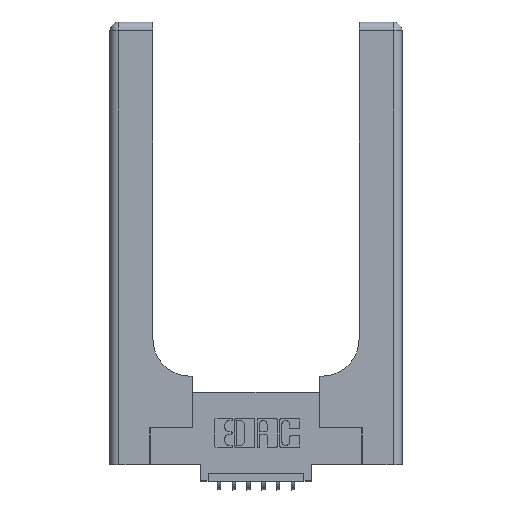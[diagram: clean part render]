
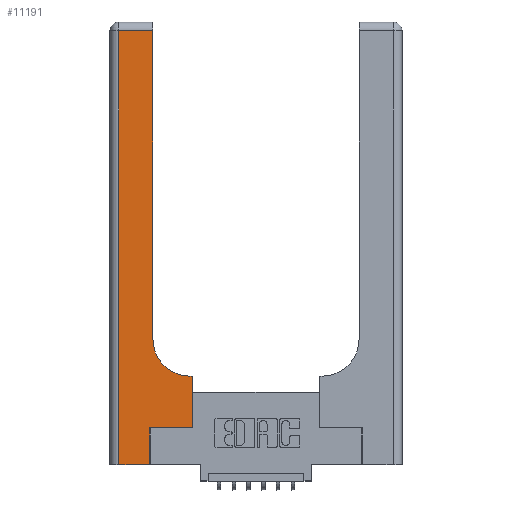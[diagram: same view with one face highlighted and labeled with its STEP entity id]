
A CAD part, top view. The second image highlights one B-rep face of the part: STEP entity #11191.
In plain terms, the highlighted planar face has unit normal (0, 0, 1).
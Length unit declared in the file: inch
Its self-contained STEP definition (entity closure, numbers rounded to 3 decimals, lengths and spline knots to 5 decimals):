
#6 = CARTESIAN_POINT ( 'NONE',  ( 0.5585, 0.6, 0.37 ) ) ;
#10 = DIRECTION ( 'NONE',  ( -1., 0., 0. ) ) ;
#196 = LINE ( 'NONE', #6288, #8931 ) ;
#241 = VECTOR ( 'NONE', #11092, 39.37008 ) ;
#779 = CARTESIAN_POINT ( 'NONE',  ( 0., 2.94, 0.37 ) ) ;
#881 = VERTEX_POINT ( 'NONE', #7257 ) ;
#1211 = DIRECTION ( 'NONE',  ( 0., 1., 0. ) ) ;
#1300 = AXIS2_PLACEMENT_3D ( 'NONE', #3464, #9089, #12483 ) ;
#1366 = CIRCLE ( 'NONE', #3056, 0.25 ) ;
#1605 = CARTESIAN_POINT ( 'NONE',  ( 0.06, 0., 0.37 ) ) ;
#1999 = ORIENTED_EDGE ( 'NONE', *, *, #5809, .T. ) ;
#2008 = VERTEX_POINT ( 'NONE', #1605 ) ;
#2251 = LINE ( 'NONE', #779, #14726 ) ;
#2322 = PLANE ( 'NONE',  #1300 ) ;
#2616 = LINE ( 'NONE', #11241, #3120 ) ;
#3010 = VERTEX_POINT ( 'NONE', #11659 ) ;
#3021 = EDGE_CURVE ( 'NONE', #881, #8735, #1366, .T. ) ;
#3056 = AXIS2_PLACEMENT_3D ( 'NONE', #10377, #7091, #3513 ) ;
#3120 = VECTOR ( 'NONE', #10, 39.37008 ) ;
#3332 = VECTOR ( 'NONE', #9706, 39.37008 ) ;
#3464 = CARTESIAN_POINT ( 'NONE',  ( 0., 3., 0.37 ) ) ;
#3513 = DIRECTION ( 'NONE',  ( 1., 0., 0. ) ) ;
#3998 = ORIENTED_EDGE ( 'NONE', *, *, #12909, .T. ) ;
#4197 = VECTOR ( 'NONE', #4644, 39.37008 ) ;
#4644 = DIRECTION ( 'NONE',  ( 0., 1., 0. ) ) ;
#4734 = LINE ( 'NONE', #7146, #4197 ) ;
#4872 = ORIENTED_EDGE ( 'NONE', *, *, #13298, .T. ) ;
#5085 = CARTESIAN_POINT ( 'NONE',  ( 0.2915, 2.94, 0.37 ) ) ;
#5089 = VECTOR ( 'NONE', #1211, 39.37008 ) ;
#5194 = ORIENTED_EDGE ( 'NONE', *, *, #3021, .T. ) ;
#5609 = EDGE_CURVE ( 'NONE', #2008, #5662, #13123, .T. ) ;
#5662 = VERTEX_POINT ( 'NONE', #8996 ) ;
#5809 = EDGE_CURVE ( 'NONE', #14651, #7820, #4734, .T. ) ;
#5838 = CARTESIAN_POINT ( 'NONE',  ( 0.2915, 3., 0.37 ) ) ;
#6124 = CARTESIAN_POINT ( 'NONE',  ( 0.5585, 0.25, 0.37 ) ) ;
#6288 = CARTESIAN_POINT ( 'NONE',  ( 0.269, 0.25, 0.37 ) ) ;
#6481 = ORIENTED_EDGE ( 'NONE', *, *, #12152, .T. ) ;
#7091 = DIRECTION ( 'NONE',  ( 0., 0., -1. ) ) ;
#7146 = CARTESIAN_POINT ( 'NONE',  ( 0.5585, 0.25, 0.37 ) ) ;
#7211 = ORIENTED_EDGE ( 'NONE', *, *, #9354, .T. ) ;
#7257 = CARTESIAN_POINT ( 'NONE',  ( 0.5415, 0.6, 0.37 ) ) ;
#7291 = EDGE_LOOP ( 'NONE', ( #6481, #7211, #8939, #11789, #4872, #3998, #1999, #8598, #5194 ) ) ;
#7618 = CARTESIAN_POINT ( 'NONE',  ( 0.2915, 0.85, 0.37 ) ) ;
#7820 = VERTEX_POINT ( 'NONE', #6 ) ;
#8059 = EDGE_CURVE ( 'NONE', #3010, #2008, #8874, .T. ) ;
#8087 = LINE ( 'NONE', #5838, #5089 ) ;
#8432 = CARTESIAN_POINT ( 'NONE',  ( 0.06, 3., 0.37 ) ) ;
#8598 = ORIENTED_EDGE ( 'NONE', *, *, #10104, .T. ) ;
#8645 = FACE_OUTER_BOUND ( 'NONE', #7291, .T. ) ;
#8735 = VERTEX_POINT ( 'NONE', #7618 ) ;
#8792 = CARTESIAN_POINT ( 'NONE',  ( 0., 0., 0.37 ) ) ;
#8815 = DIRECTION ( 'NONE',  ( -1., 0., 0. ) ) ;
#8874 = LINE ( 'NONE', #8432, #3332 ) ;
#8931 = VECTOR ( 'NONE', #9494, 39.37008 ) ;
#8939 = ORIENTED_EDGE ( 'NONE', *, *, #8059, .T. ) ;
#8996 = CARTESIAN_POINT ( 'NONE',  ( 0.269, 0., 0.37 ) ) ;
#9089 = DIRECTION ( 'NONE',  ( 0., 0., -1. ) ) ;
#9354 = EDGE_CURVE ( 'NONE', #13551, #3010, #2251, .T. ) ;
#9379 = CARTESIAN_POINT ( 'NONE',  ( 0.269, 0., 0.37 ) ) ;
#9494 = DIRECTION ( 'NONE',  ( 1., 0., 0. ) ) ;
#9706 = DIRECTION ( 'NONE',  ( 0., -1., 0. ) ) ;
#9979 = CARTESIAN_POINT ( 'NONE',  ( 0.269, 0.25, 0.37 ) ) ;
#10104 = EDGE_CURVE ( 'NONE', #7820, #881, #2616, .T. ) ;
#10377 = CARTESIAN_POINT ( 'NONE',  ( 0.5415, 0.85, 0.37 ) ) ;
#11092 = DIRECTION ( 'NONE',  ( 1., 0., 0. ) ) ;
#11191 = ADVANCED_FACE ( 'NONE', ( #8645 ), #2322, .F. ) ;
#11241 = CARTESIAN_POINT ( 'NONE',  ( 0.2915, 0.6, 0.37 ) ) ;
#11527 = DIRECTION ( 'NONE',  ( 0., 1., 0. ) ) ;
#11622 = LINE ( 'NONE', #9379, #13754 ) ;
#11659 = CARTESIAN_POINT ( 'NONE',  ( 0.06, 2.94, 0.37 ) ) ;
#11789 = ORIENTED_EDGE ( 'NONE', *, *, #5609, .T. ) ;
#12054 = VERTEX_POINT ( 'NONE', #9979 ) ;
#12152 = EDGE_CURVE ( 'NONE', #8735, #13551, #8087, .T. ) ;
#12483 = DIRECTION ( 'NONE',  ( -1., 0., 0. ) ) ;
#12909 = EDGE_CURVE ( 'NONE', #12054, #14651, #196, .T. ) ;
#13123 = LINE ( 'NONE', #8792, #241 ) ;
#13298 = EDGE_CURVE ( 'NONE', #5662, #12054, #11622, .T. ) ;
#13551 = VERTEX_POINT ( 'NONE', #5085 ) ;
#13754 = VECTOR ( 'NONE', #11527, 39.37008 ) ;
#14651 = VERTEX_POINT ( 'NONE', #6124 ) ;
#14726 = VECTOR ( 'NONE', #8815, 39.37008 ) ;
